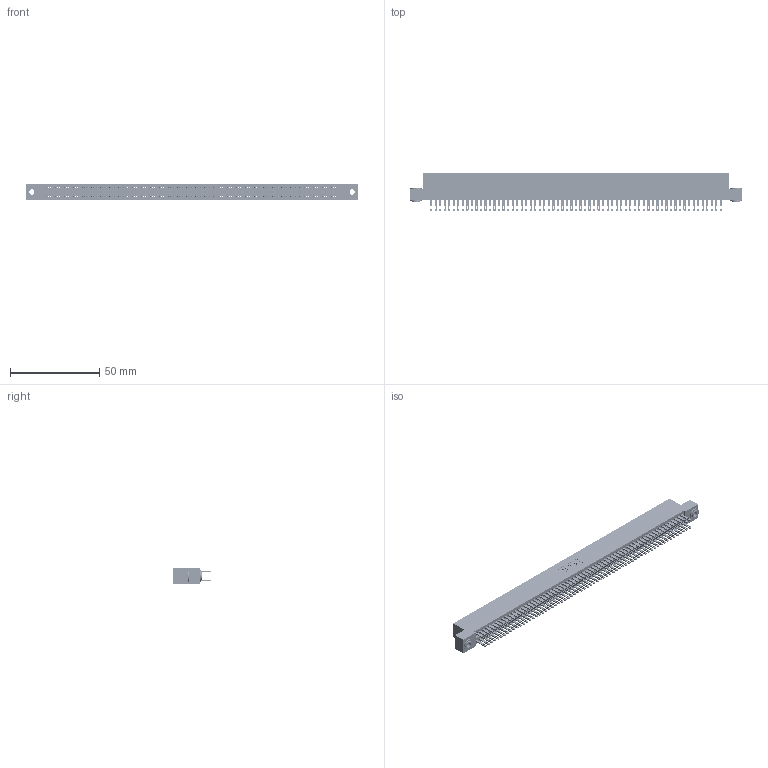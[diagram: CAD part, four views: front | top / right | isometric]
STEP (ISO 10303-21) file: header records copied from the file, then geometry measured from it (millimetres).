
FILE_DESCRIPTION (( 'STEP AP203' ), '1' );
FILE_NAME ('345-130-500-203.STEP', '2019-11-07T11:25:16', ( '' ), ( '' ), 'SwSTEP 2.0', 'SolidWorks 2016', '' );
FILE_SCHEMA (( 'CONFIG_CONTROL_DESIGN' ));
Length unit declared in the file: inch
Products named in the file (4): 345 Part_Flush Mounting Lugs - 0.156 Dia-TH; 345-250-002_345-250-002-102; 345-292-001_345-293-100; 345-130-500-203
Assembly tree (133 placements, depth 2):
  345-130-500-203
    345 Part_Flush Mounting Lugs - 0.156 Dia-TH
    345-292-001_345-293-100  x130
    345-250-002_345-250-002-102  x2
Bounding box: 186.31 x 21.51 x 9.4 mm (x, y, z)
Volume: 18728.4 mm3; surface area: 29660 mm2
Topology: 133 solids, 133 shells, 6144 faces, 18747 edges, 12494 vertices
Faces by surface type: plane 3600, cylinder 2536, cone 8
Entity records: 48484 total; most frequent: CARTESIAN_POINT 8079, ORIENTED_EDGE 8006, DIRECTION 7129, EDGE_CURVE 4003, VECTOR 3583, LINE 3583, VERTEX_POINT 2666, AXIS2_PLACEMENT_3D 1773
